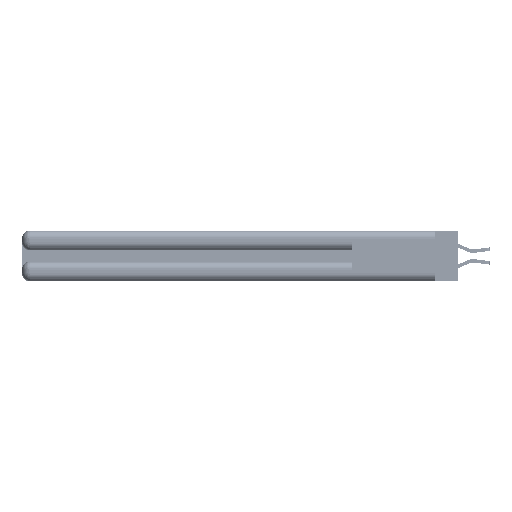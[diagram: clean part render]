
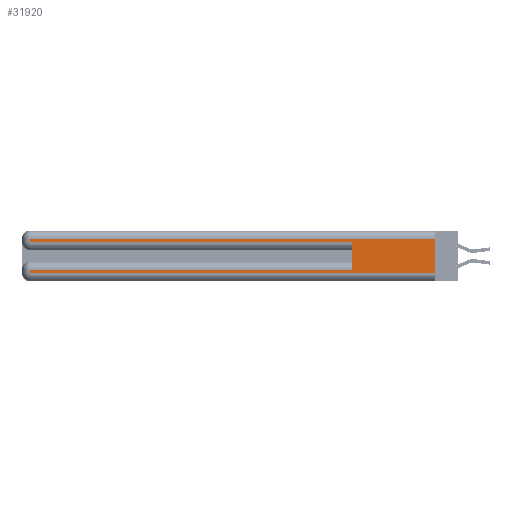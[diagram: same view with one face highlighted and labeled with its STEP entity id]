
A CAD part, left-side view. The second image highlights one B-rep face of the part: STEP entity #31920.
In plain terms, the highlighted planar face has unit normal (-1, 0, 0).
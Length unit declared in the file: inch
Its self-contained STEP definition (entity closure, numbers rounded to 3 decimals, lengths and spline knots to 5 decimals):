
#146 = VERTEX_POINT ( 'NONE', #3165 ) ;
#242 = CARTESIAN_POINT ( 'NONE',  ( 0., 0.6, 0.085 ) ) ;
#245 = VECTOR ( 'NONE', #27757, 39.37008 ) ;
#597 = VERTEX_POINT ( 'NONE', #27797 ) ;
#1041 = EDGE_CURVE ( 'NONE', #597, #18590, #36664, .T. ) ;
#1255 = LINE ( 'NONE', #27585, #245 ) ;
#1274 = VECTOR ( 'NONE', #39508, 39.37008 ) ;
#1404 = PLANE ( 'NONE',  #26356 ) ;
#2081 = CARTESIAN_POINT ( 'NONE',  ( 0., 0., 0.06 ) ) ;
#2139 = EDGE_CURVE ( 'NONE', #21933, #25339, #2706, .T. ) ;
#2658 = DIRECTION ( 'NONE',  ( 0., 0., -1. ) ) ;
#2706 = LINE ( 'NONE', #26630, #18660 ) ;
#3165 = CARTESIAN_POINT ( 'NONE',  ( 0., 2.94, 0.285 ) ) ;
#3351 = DIRECTION ( 'NONE',  ( 0., -1., 0. ) ) ;
#4390 = EDGE_CURVE ( 'NONE', #25339, #10871, #34947, .T. ) ;
#4813 = CARTESIAN_POINT ( 'NONE',  ( 0., 0., 0.06 ) ) ;
#5298 = FACE_OUTER_BOUND ( 'NONE', #7352, .T. ) ;
#6145 = CARTESIAN_POINT ( 'NONE',  ( 0., 0.6, 0.285 ) ) ;
#7352 = EDGE_LOOP ( 'NONE', ( #37571, #27200, #26692, #37722, #9054, #36502, #9289, #40263 ) ) ;
#7409 = VECTOR ( 'NONE', #2658, 39.37008 ) ;
#7746 = CARTESIAN_POINT ( 'NONE',  ( 0., 2.94, 0.06 ) ) ;
#9054 = ORIENTED_EDGE ( 'NONE', *, *, #25574, .F. ) ;
#9289 = ORIENTED_EDGE ( 'NONE', *, *, #2139, .T. ) ;
#9364 = EDGE_CURVE ( 'NONE', #18590, #146, #16941, .T. ) ;
#9501 = CARTESIAN_POINT ( 'NONE',  ( 0., 2.94, 0.085 ) ) ;
#9614 = LINE ( 'NONE', #15447, #17639 ) ;
#10199 = CARTESIAN_POINT ( 'NONE',  ( 0., 0., 0.31 ) ) ;
#10871 = VERTEX_POINT ( 'NONE', #2081 ) ;
#10917 = LINE ( 'NONE', #11904, #7409 ) ;
#11904 = CARTESIAN_POINT ( 'NONE',  ( 0., 0., 0.37 ) ) ;
#11933 = CARTESIAN_POINT ( 'NONE',  ( 0., 2.94, 0.31 ) ) ;
#13272 = VECTOR ( 'NONE', #3351, 39.37008 ) ;
#14058 = EDGE_CURVE ( 'NONE', #597, #10871, #10917, .T. ) ;
#14603 = DIRECTION ( 'NONE',  ( 1., 0., 0. ) ) ;
#15447 = CARTESIAN_POINT ( 'NONE',  ( 0., 0.6, 0.145 ) ) ;
#16941 = LINE ( 'NONE', #37395, #40822 ) ;
#17639 = VECTOR ( 'NONE', #37768, 39.37008 ) ;
#17685 = EDGE_CURVE ( 'NONE', #32350, #21933, #1255, .T. ) ;
#18590 = VERTEX_POINT ( 'NONE', #11933 ) ;
#18660 = VECTOR ( 'NONE', #21511, 39.37008 ) ;
#21511 = DIRECTION ( 'NONE',  ( 0., 0., -1. ) ) ;
#21933 = VERTEX_POINT ( 'NONE', #9501 ) ;
#22361 = CARTESIAN_POINT ( 'NONE',  ( 0., 0., 0.285 ) ) ;
#23506 = VECTOR ( 'NONE', #30419, 39.37008 ) ;
#23597 = VERTEX_POINT ( 'NONE', #6145 ) ;
#24335 = LINE ( 'NONE', #22361, #13272 ) ;
#25339 = VERTEX_POINT ( 'NONE', #7746 ) ;
#25574 = EDGE_CURVE ( 'NONE', #32350, #23597, #9614, .T. ) ;
#26356 = AXIS2_PLACEMENT_3D ( 'NONE', #36786, #14603, #33844 ) ;
#26630 = CARTESIAN_POINT ( 'NONE',  ( 0., 2.94, 0.37 ) ) ;
#26692 = ORIENTED_EDGE ( 'NONE', *, *, #9364, .T. ) ;
#27200 = ORIENTED_EDGE ( 'NONE', *, *, #1041, .T. ) ;
#27585 = CARTESIAN_POINT ( 'NONE',  ( 0., 0., 0.085 ) ) ;
#27757 = DIRECTION ( 'NONE',  ( 0., 1., 0. ) ) ;
#27797 = CARTESIAN_POINT ( 'NONE',  ( 0., 0., 0.31 ) ) ;
#29332 = EDGE_CURVE ( 'NONE', #146, #23597, #24335, .T. ) ;
#30419 = DIRECTION ( 'NONE',  ( 0., -1., 0. ) ) ;
#31920 = ADVANCED_FACE ( 'NONE', ( #5298 ), #1404, .F. ) ;
#32350 = VERTEX_POINT ( 'NONE', #242 ) ;
#33844 = DIRECTION ( 'NONE',  ( 0., 0., -1. ) ) ;
#34947 = LINE ( 'NONE', #4813, #23506 ) ;
#36502 = ORIENTED_EDGE ( 'NONE', *, *, #17685, .T. ) ;
#36664 = LINE ( 'NONE', #10199, #1274 ) ;
#36786 = CARTESIAN_POINT ( 'NONE',  ( 0., 0., 0.37 ) ) ;
#37395 = CARTESIAN_POINT ( 'NONE',  ( 0., 2.94, 0.37 ) ) ;
#37571 = ORIENTED_EDGE ( 'NONE', *, *, #14058, .F. ) ;
#37722 = ORIENTED_EDGE ( 'NONE', *, *, #29332, .T. ) ;
#37768 = DIRECTION ( 'NONE',  ( 0., 0., 1. ) ) ;
#39508 = DIRECTION ( 'NONE',  ( 0., 1., 0. ) ) ;
#40263 = ORIENTED_EDGE ( 'NONE', *, *, #4390, .T. ) ;
#40547 = DIRECTION ( 'NONE',  ( 0., 0., -1. ) ) ;
#40822 = VECTOR ( 'NONE', #40547, 39.37008 ) ;
